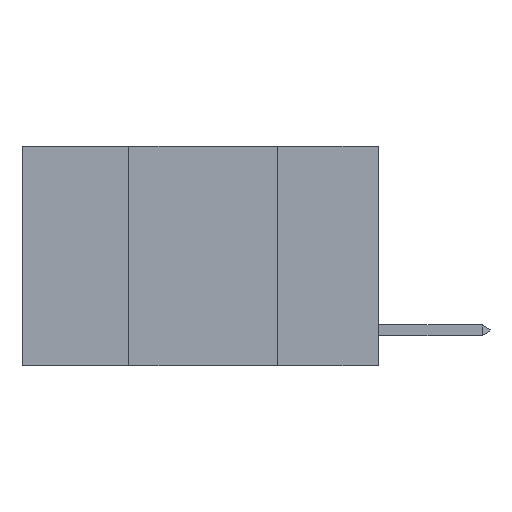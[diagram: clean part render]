
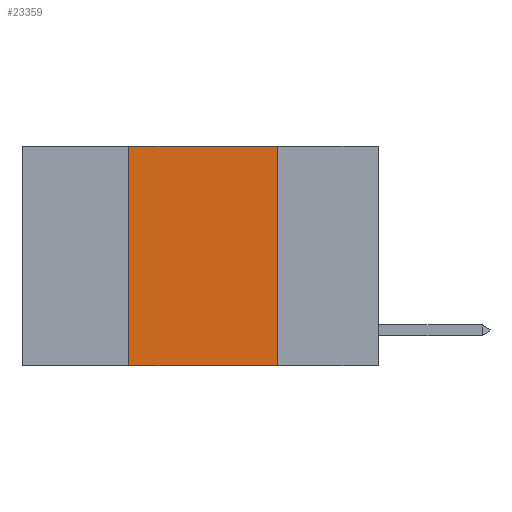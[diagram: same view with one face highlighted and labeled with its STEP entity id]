
A CAD part, left-side view. The second image highlights one B-rep face of the part: STEP entity #23359.
In plain terms, the highlighted planar face has unit normal (-1, 0, 0).
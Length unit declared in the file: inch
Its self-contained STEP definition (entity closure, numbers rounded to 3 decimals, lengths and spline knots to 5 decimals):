
#501 = AXIS2_PLACEMENT_3D ( 'NONE', #15032, #1383, #17347 ) ;
#1383 = DIRECTION ( 'NONE',  ( 1., 0., 0. ) ) ;
#2755 = DIRECTION ( 'NONE',  ( 0., 0., -1. ) ) ;
#3206 = CARTESIAN_POINT ( 'NONE',  ( 0., 0.6, 0. ) ) ;
#4463 = CARTESIAN_POINT ( 'NONE',  ( 0., 0.42, -0.37 ) ) ;
#5398 = VECTOR ( 'NONE', #21445, 39.37008 ) ;
#6754 = CARTESIAN_POINT ( 'NONE',  ( 0., 0.42, 0. ) ) ;
#7820 = CARTESIAN_POINT ( 'NONE',  ( 0., 0.6, -0.37 ) ) ;
#7909 = EDGE_CURVE ( 'NONE', #16298, #27272, #24762, .T. ) ;
#8896 = VECTOR ( 'NONE', #15461, 39.37008 ) ;
#10359 = LINE ( 'NONE', #16477, #22455 ) ;
#13759 = ORIENTED_EDGE ( 'NONE', *, *, #20447, .F. ) ;
#15016 = CARTESIAN_POINT ( 'NONE',  ( 0., 0.17, 0. ) ) ;
#15031 = LINE ( 'NONE', #20032, #8896 ) ;
#15032 = CARTESIAN_POINT ( 'NONE',  ( 0., 0.6, 0. ) ) ;
#15461 = DIRECTION ( 'NONE',  ( 0., 0., 1. ) ) ;
#15684 = EDGE_CURVE ( 'NONE', #16298, #28624, #15031, .T. ) ;
#15976 = ORIENTED_EDGE ( 'NONE', *, *, #7909, .T. ) ;
#16298 = VERTEX_POINT ( 'NONE', #4463 ) ;
#16477 = CARTESIAN_POINT ( 'NONE',  ( 0., 0.17, 0. ) ) ;
#17347 = DIRECTION ( 'NONE',  ( 0., 0., -1. ) ) ;
#18586 = VERTEX_POINT ( 'NONE', #15016 ) ;
#19502 = VECTOR ( 'NONE', #23794, 39.37008 ) ;
#20032 = CARTESIAN_POINT ( 'NONE',  ( 0., 0.42, 0. ) ) ;
#20447 = EDGE_CURVE ( 'NONE', #28624, #18586, #24314, .T. ) ;
#20632 = FACE_OUTER_BOUND ( 'NONE', #28098, .T. ) ;
#21445 = DIRECTION ( 'NONE',  ( 0., -1., 0. ) ) ;
#21712 = EDGE_CURVE ( 'NONE', #18586, #27272, #10359, .T. ) ;
#21769 = PLANE ( 'NONE',  #501 ) ;
#22455 = VECTOR ( 'NONE', #2755, 39.37008 ) ;
#23359 = ADVANCED_FACE ( 'NONE', ( #20632 ), #21769, .F. ) ;
#23794 = DIRECTION ( 'NONE',  ( 0., -1., 0. ) ) ;
#24314 = LINE ( 'NONE', #3206, #5398 ) ;
#24762 = LINE ( 'NONE', #7820, #19502 ) ;
#25364 = CARTESIAN_POINT ( 'NONE',  ( 0., 0.17, -0.37 ) ) ;
#25806 = ORIENTED_EDGE ( 'NONE', *, *, #21712, .F. ) ;
#27272 = VERTEX_POINT ( 'NONE', #25364 ) ;
#28098 = EDGE_LOOP ( 'NONE', ( #25806, #13759, #28189, #15976 ) ) ;
#28189 = ORIENTED_EDGE ( 'NONE', *, *, #15684, .F. ) ;
#28624 = VERTEX_POINT ( 'NONE', #6754 ) ;
